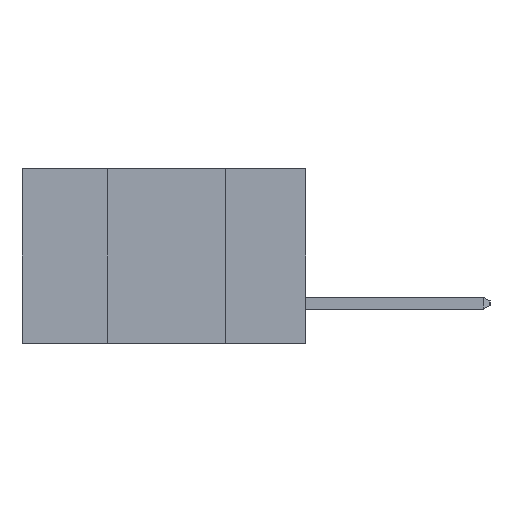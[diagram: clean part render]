
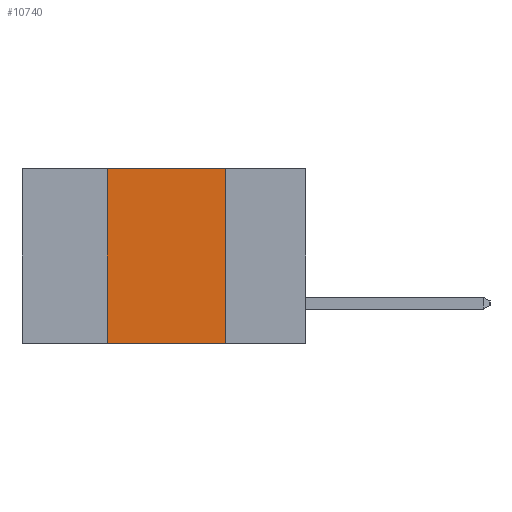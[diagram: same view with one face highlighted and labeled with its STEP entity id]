
A CAD part, left-side view. The second image highlights one B-rep face of the part: STEP entity #10740.
In plain terms, the highlighted planar face has unit normal (-1, 0, 0).
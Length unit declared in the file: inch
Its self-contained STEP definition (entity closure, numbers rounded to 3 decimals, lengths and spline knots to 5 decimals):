
#117 = ORIENTED_EDGE ( 'NONE', *, *, #8210, .F. ) ;
#202 = ORIENTED_EDGE ( 'NONE', *, *, #14295, .F. ) ;
#233 = ORIENTED_EDGE ( 'NONE', *, *, #13309, .F. ) ;
#295 = ORIENTED_EDGE ( 'NONE', *, *, #9317, .T. ) ;
#358 = CARTESIAN_POINT ( 'NONE',  ( 0., 0.6, 0. ) ) ;
#981 = AXIS2_PLACEMENT_3D ( 'NONE', #7187, #4666, #13449 ) ;
#2258 = VERTEX_POINT ( 'NONE', #11883 ) ;
#2509 = VERTEX_POINT ( 'NONE', #15510 ) ;
#2737 = LINE ( 'NONE', #14729, #6146 ) ;
#3133 = VECTOR ( 'NONE', #14453, 39.37008 ) ;
#3447 = DIRECTION ( 'NONE',  ( 0., 0., 1. ) ) ;
#3579 = EDGE_LOOP ( 'NONE', ( #117, #202, #233, #295 ) ) ;
#3682 = VECTOR ( 'NONE', #8316, 39.37008 ) ;
#4666 = DIRECTION ( 'NONE',  ( 1., 0., 0. ) ) ;
#6146 = VECTOR ( 'NONE', #3447, 39.37008 ) ;
#7187 = CARTESIAN_POINT ( 'NONE',  ( 0., 0.6, 0. ) ) ;
#8005 = DIRECTION ( 'NONE',  ( 0., -1., 0. ) ) ;
#8030 = FACE_OUTER_BOUND ( 'NONE', #3579, .T. ) ;
#8210 = EDGE_CURVE ( 'NONE', #2509, #11152, #13223, .T. ) ;
#8316 = DIRECTION ( 'NONE',  ( 0., -1., 0. ) ) ;
#9317 = EDGE_CURVE ( 'NONE', #9599, #11152, #13761, .T. ) ;
#9599 = VERTEX_POINT ( 'NONE', #14925 ) ;
#9659 = CARTESIAN_POINT ( 'NONE',  ( 0., 0.6, -0.37 ) ) ;
#10519 = VECTOR ( 'NONE', #8005, 39.37008 ) ;
#10740 = ADVANCED_FACE ( 'NONE', ( #8030 ), #12269, .F. ) ;
#11152 = VERTEX_POINT ( 'NONE', #14232 ) ;
#11883 = CARTESIAN_POINT ( 'NONE',  ( 0., 0.42, 0. ) ) ;
#12269 = PLANE ( 'NONE',  #981 ) ;
#13223 = LINE ( 'NONE', #15263, #3133 ) ;
#13309 = EDGE_CURVE ( 'NONE', #9599, #2258, #2737, .T. ) ;
#13449 = DIRECTION ( 'NONE',  ( 0., 0., -1. ) ) ;
#13761 = LINE ( 'NONE', #9659, #3682 ) ;
#14232 = CARTESIAN_POINT ( 'NONE',  ( 0., 0.17, -0.37 ) ) ;
#14295 = EDGE_CURVE ( 'NONE', #2258, #2509, #16150, .T. ) ;
#14453 = DIRECTION ( 'NONE',  ( 0., 0., -1. ) ) ;
#14729 = CARTESIAN_POINT ( 'NONE',  ( 0., 0.42, -0.37 ) ) ;
#14925 = CARTESIAN_POINT ( 'NONE',  ( 0., 0.42, -0.37 ) ) ;
#15263 = CARTESIAN_POINT ( 'NONE',  ( 0., 0.17, -0.37 ) ) ;
#15510 = CARTESIAN_POINT ( 'NONE',  ( 0., 0.17, 0. ) ) ;
#16150 = LINE ( 'NONE', #358, #10519 ) ;
